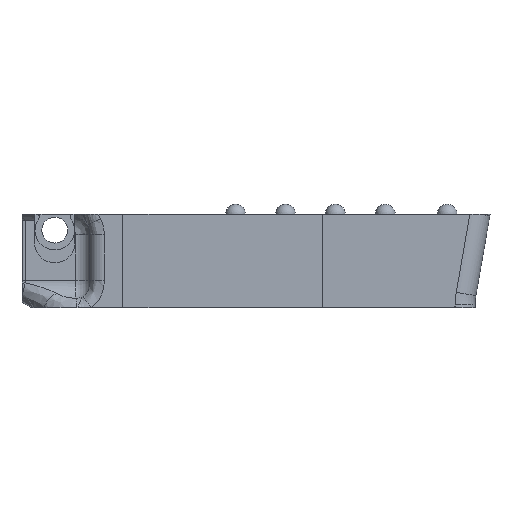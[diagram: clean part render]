
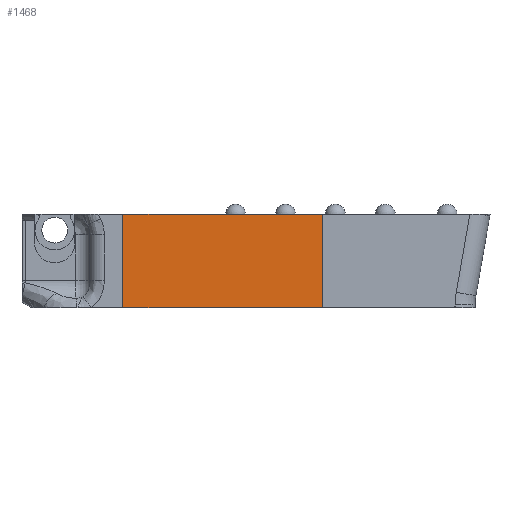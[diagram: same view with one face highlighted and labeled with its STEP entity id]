
A CAD part, front view. The second image highlights one B-rep face of the part: STEP entity #1468.
In plain terms, the highlighted planar face has unit normal (0, -1, 0).
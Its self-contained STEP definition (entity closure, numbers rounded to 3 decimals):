
#208 = DIRECTION ( 'NONE',  ( 0., -1., 0. ) ) ;
#258 = CARTESIAN_POINT ( 'NONE',  ( 0., -47.207, -5.481 ) ) ;
#824 = EDGE_CURVE ( 'NONE', #2165, #1322, #3682, .T. ) ;
#881 = CARTESIAN_POINT ( 'NONE',  ( 142.429, -47.207, -5.481 ) ) ;
#1298 = PLANE ( 'NONE',  #1704 ) ;
#1310 = CARTESIAN_POINT ( 'NONE',  ( 102.429, -47.207, -5.481 ) ) ;
#1322 = VERTEX_POINT ( 'NONE', #4592 ) ;
#1362 = CARTESIAN_POINT ( 'NONE',  ( 142.429, -47.207, 13.231 ) ) ;
#1468 = ADVANCED_FACE ( 'NONE', ( #1554 ), #1298, .T. ) ;
#1554 = FACE_OUTER_BOUND ( 'NONE', #3896, .T. ) ;
#1704 = AXIS2_PLACEMENT_3D ( 'NONE', #2350, #208, #4133 ) ;
#1771 = DIRECTION ( 'NONE',  ( 0., 0., 1. ) ) ;
#1790 = LINE ( 'NONE', #2869, #3739 ) ;
#1867 = DIRECTION ( 'NONE',  ( -1., 0., 0. ) ) ;
#1967 = EDGE_CURVE ( 'NONE', #3866, #3758, #3895, .T. ) ;
#2050 = EDGE_CURVE ( 'NONE', #3758, #2165, #2447, .T. ) ;
#2165 = VERTEX_POINT ( 'NONE', #1362 ) ;
#2350 = CARTESIAN_POINT ( 'NONE',  ( 0., -47.207, 0. ) ) ;
#2447 = LINE ( 'NONE', #3941, #4574 ) ;
#2476 = DIRECTION ( 'NONE',  ( 1., 0., 0. ) ) ;
#2853 = EDGE_CURVE ( 'NONE', #1322, #3866, #1790, .T. ) ;
#2869 = CARTESIAN_POINT ( 'NONE',  ( 102.429, -47.207, 0. ) ) ;
#3047 = ORIENTED_EDGE ( 'NONE', *, *, #1967, .T. ) ;
#3054 = VECTOR ( 'NONE', #2476, 1000. ) ;
#3166 = ORIENTED_EDGE ( 'NONE', *, *, #2050, .T. ) ;
#3519 = ORIENTED_EDGE ( 'NONE', *, *, #824, .T. ) ;
#3560 = DIRECTION ( 'NONE',  ( 0., 0., -1. ) ) ;
#3682 = LINE ( 'NONE', #3722, #4071 ) ;
#3722 = CARTESIAN_POINT ( 'NONE',  ( 0., -47.207, 13.231 ) ) ;
#3739 = VECTOR ( 'NONE', #3560, 1000. ) ;
#3758 = VERTEX_POINT ( 'NONE', #881 ) ;
#3855 = ORIENTED_EDGE ( 'NONE', *, *, #2853, .T. ) ;
#3866 = VERTEX_POINT ( 'NONE', #1310 ) ;
#3895 = LINE ( 'NONE', #258, #3054 ) ;
#3896 = EDGE_LOOP ( 'NONE', ( #3519, #3855, #3047, #3166 ) ) ;
#3941 = CARTESIAN_POINT ( 'NONE',  ( 142.429, -47.207, 0. ) ) ;
#4071 = VECTOR ( 'NONE', #1867, 1000. ) ;
#4133 = DIRECTION ( 'NONE',  ( 0., 0., -1. ) ) ;
#4574 = VECTOR ( 'NONE', #1771, 1000. ) ;
#4592 = CARTESIAN_POINT ( 'NONE',  ( 102.429, -47.207, 13.231 ) ) ;
